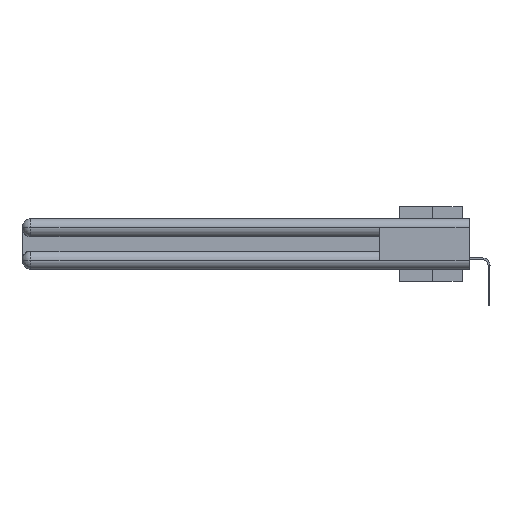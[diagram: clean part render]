
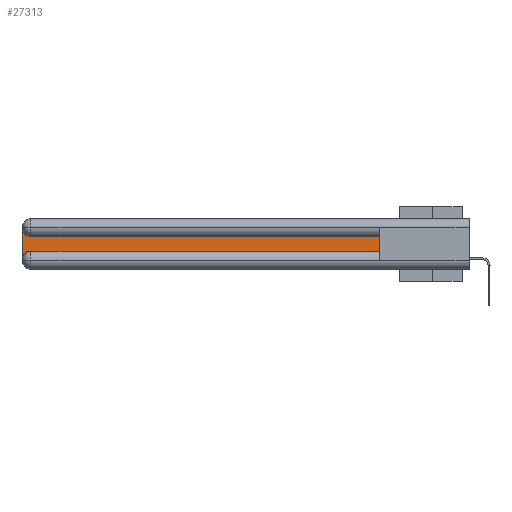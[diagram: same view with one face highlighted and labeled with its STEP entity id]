
A CAD part, left-side view. The second image highlights one B-rep face of the part: STEP entity #27313.
In plain terms, the highlighted planar face has unit normal (-1, 0, 0).
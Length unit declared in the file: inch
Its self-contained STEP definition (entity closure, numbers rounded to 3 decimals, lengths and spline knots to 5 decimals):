
#1121 = EDGE_CURVE ( 'NONE', #7447, #6782, #30808, .T. ) ;
#2121 = ORIENTED_EDGE ( 'NONE', *, *, #5671, .T. ) ;
#2147 = AXIS2_PLACEMENT_3D ( 'NONE', #24450, #26950, #15894 ) ;
#2599 = DIRECTION ( 'NONE',  ( 0., 0., -1. ) ) ;
#2982 = VERTEX_POINT ( 'NONE', #26686 ) ;
#3107 = EDGE_CURVE ( 'NONE', #36751, #16976, #8054, .T. ) ;
#4462 = LINE ( 'NONE', #8751, #26495 ) ;
#5671 = EDGE_CURVE ( 'NONE', #6782, #36751, #18193, .T. ) ;
#5764 = FACE_OUTER_BOUND ( 'NONE', #10280, .T. ) ;
#6744 = ORIENTED_EDGE ( 'NONE', *, *, #20264, .T. ) ;
#6782 = VERTEX_POINT ( 'NONE', #20904 ) ;
#7447 = VERTEX_POINT ( 'NONE', #32562 ) ;
#8054 = LINE ( 'NONE', #9853, #27871 ) ;
#8751 = CARTESIAN_POINT ( 'NONE',  ( 0.075, 0.6, -0.1225 ) ) ;
#8971 = CARTESIAN_POINT ( 'NONE',  ( 0.075, 3., -0.1225 ) ) ;
#9243 = AXIS2_PLACEMENT_3D ( 'NONE', #24696, #18560, #18674 ) ;
#9853 = CARTESIAN_POINT ( 'NONE',  ( 0.075, 0.6, -0.2175 ) ) ;
#10280 = EDGE_LOOP ( 'NONE', ( #6744, #29937, #34084, #12338, #2121, #13161 ) ) ;
#12231 = DIRECTION ( 'NONE',  ( 0., 0., -1. ) ) ;
#12338 = ORIENTED_EDGE ( 'NONE', *, *, #1121, .T. ) ;
#13161 = ORIENTED_EDGE ( 'NONE', *, *, #3107, .T. ) ;
#13249 = CARTESIAN_POINT ( 'NONE',  ( 0.075, 3., -0.0625 ) ) ;
#15013 = DIRECTION ( 'NONE',  ( 1., 0., 0. ) ) ;
#15300 = EDGE_CURVE ( 'NONE', #31872, #7447, #17809, .T. ) ;
#15894 = DIRECTION ( 'NONE',  ( 0., 0., -1. ) ) ;
#16976 = VERTEX_POINT ( 'NONE', #36191 ) ;
#17809 = LINE ( 'NONE', #19686, #32180 ) ;
#18193 = LINE ( 'NONE', #19571, #25385 ) ;
#18560 = DIRECTION ( 'NONE',  ( 1., 0., 0. ) ) ;
#18674 = DIRECTION ( 'NONE',  ( 0., 0., -1. ) ) ;
#19571 = CARTESIAN_POINT ( 'NONE',  ( 0.075, 0.6, -0.2175 ) ) ;
#19686 = CARTESIAN_POINT ( 'NONE',  ( 0.075, 3., -0.2175 ) ) ;
#20264 = EDGE_CURVE ( 'NONE', #16976, #2982, #4462, .T. ) ;
#20426 = PLANE ( 'NONE',  #34330 ) ;
#20495 = EDGE_CURVE ( 'NONE', #2982, #31872, #29186, .T. ) ;
#20904 = CARTESIAN_POINT ( 'NONE',  ( 0.075, 2.94, -0.2175 ) ) ;
#21178 = DIRECTION ( 'NONE',  ( 0., 0., 1. ) ) ;
#23957 = CARTESIAN_POINT ( 'NONE',  ( 0.075, 0.6, -0.2175 ) ) ;
#24450 = CARTESIAN_POINT ( 'NONE',  ( 0.075, 2.94, -0.0625 ) ) ;
#24696 = CARTESIAN_POINT ( 'NONE',  ( 0.075, 2.94, -0.2775 ) ) ;
#25385 = VECTOR ( 'NONE', #28380, 39.37008 ) ;
#26451 = DIRECTION ( 'NONE',  ( 0., 1., 0. ) ) ;
#26495 = VECTOR ( 'NONE', #26451, 39.37008 ) ;
#26686 = CARTESIAN_POINT ( 'NONE',  ( 0.075, 2.94, -0.1225 ) ) ;
#26950 = DIRECTION ( 'NONE',  ( 1., 0., 0. ) ) ;
#27313 = ADVANCED_FACE ( 'NONE', ( #5764 ), #20426, .F. ) ;
#27871 = VECTOR ( 'NONE', #21178, 39.37008 ) ;
#28380 = DIRECTION ( 'NONE',  ( 0., -1., 0. ) ) ;
#29186 = CIRCLE ( 'NONE', #2147, 0.06 ) ;
#29937 = ORIENTED_EDGE ( 'NONE', *, *, #20495, .T. ) ;
#30808 = CIRCLE ( 'NONE', #9243, 0.06 ) ;
#31872 = VERTEX_POINT ( 'NONE', #13249 ) ;
#32180 = VECTOR ( 'NONE', #2599, 39.37008 ) ;
#32562 = CARTESIAN_POINT ( 'NONE',  ( 0.075, 3., -0.2775 ) ) ;
#34084 = ORIENTED_EDGE ( 'NONE', *, *, #15300, .T. ) ;
#34330 = AXIS2_PLACEMENT_3D ( 'NONE', #8971, #15013, #12231 ) ;
#36191 = CARTESIAN_POINT ( 'NONE',  ( 0.075, 0.6, -0.1225 ) ) ;
#36751 = VERTEX_POINT ( 'NONE', #23957 ) ;
